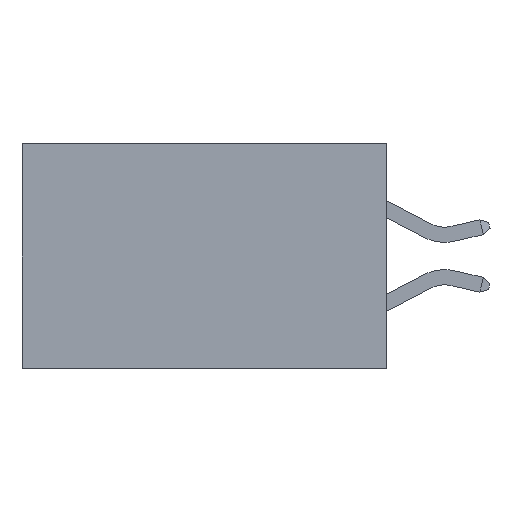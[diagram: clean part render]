
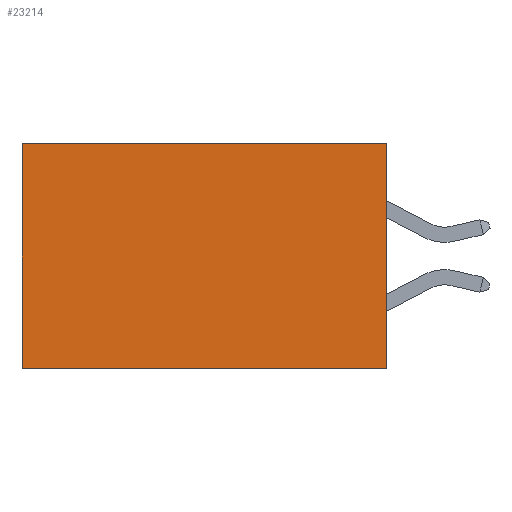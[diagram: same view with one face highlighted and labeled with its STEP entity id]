
A CAD part, left-side view. The second image highlights one B-rep face of the part: STEP entity #23214.
In plain terms, the highlighted planar face has unit normal (-1, 0, 0).
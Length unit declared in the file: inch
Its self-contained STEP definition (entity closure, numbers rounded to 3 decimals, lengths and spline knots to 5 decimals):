
#8 = CARTESIAN_POINT ( 'NONE',  ( 0.2615, 0.6, 0. ) ) ;
#512 = EDGE_CURVE ( 'NONE', #2261, #23418, #26246, .T. ) ;
#736 = DIRECTION ( 'NONE',  ( 0., 0., -1. ) ) ;
#1049 = ORIENTED_EDGE ( 'NONE', *, *, #23925, .T. ) ;
#1179 = ORIENTED_EDGE ( 'NONE', *, *, #15550, .T. ) ;
#2261 = VERTEX_POINT ( 'NONE', #14005 ) ;
#2907 = VECTOR ( 'NONE', #22642, 39.37008 ) ;
#3391 = CARTESIAN_POINT ( 'NONE',  ( 0.2615, 0.6, -0.37 ) ) ;
#4437 = CARTESIAN_POINT ( 'NONE',  ( 0.2615, 0., -0.37 ) ) ;
#4518 = CARTESIAN_POINT ( 'NONE',  ( 0.2615, 0., -0.37 ) ) ;
#5693 = EDGE_CURVE ( 'NONE', #11454, #2261, #9835, .T. ) ;
#6602 = DIRECTION ( 'NONE',  ( 0., 0., -1. ) ) ;
#8144 = VECTOR ( 'NONE', #21657, 39.37008 ) ;
#9596 = VECTOR ( 'NONE', #12702, 39.37008 ) ;
#9835 = LINE ( 'NONE', #4437, #14588 ) ;
#10868 = VERTEX_POINT ( 'NONE', #8 ) ;
#11454 = VERTEX_POINT ( 'NONE', #26179 ) ;
#12702 = DIRECTION ( 'NONE',  ( 0., 1., 0. ) ) ;
#13199 = DIRECTION ( 'NONE',  ( 1., 0., 0. ) ) ;
#13914 = LINE ( 'NONE', #20585, #2907 ) ;
#14005 = CARTESIAN_POINT ( 'NONE',  ( 0.2615, 0., -0.37 ) ) ;
#14588 = VECTOR ( 'NONE', #6602, 39.37008 ) ;
#15148 = PLANE ( 'NONE',  #22758 ) ;
#15550 = EDGE_CURVE ( 'NONE', #11454, #10868, #13914, .T. ) ;
#17703 = ORIENTED_EDGE ( 'NONE', *, *, #5693, .F. ) ;
#18888 = EDGE_LOOP ( 'NONE', ( #1049, #23483, #17703, #1179 ) ) ;
#19605 = CARTESIAN_POINT ( 'NONE',  ( 0.2615, 0.6, -0.37 ) ) ;
#20585 = CARTESIAN_POINT ( 'NONE',  ( 0.2615, 0., 0. ) ) ;
#21657 = DIRECTION ( 'NONE',  ( 0., 0., -1. ) ) ;
#22642 = DIRECTION ( 'NONE',  ( 0., 1., 0. ) ) ;
#22758 = AXIS2_PLACEMENT_3D ( 'NONE', #25232, #13199, #736 ) ;
#23214 = ADVANCED_FACE ( 'NONE', ( #24601 ), #15148, .F. ) ;
#23418 = VERTEX_POINT ( 'NONE', #3391 ) ;
#23483 = ORIENTED_EDGE ( 'NONE', *, *, #512, .F. ) ;
#23925 = EDGE_CURVE ( 'NONE', #10868, #23418, #24230, .T. ) ;
#24230 = LINE ( 'NONE', #19605, #8144 ) ;
#24601 = FACE_OUTER_BOUND ( 'NONE', #18888, .T. ) ;
#25232 = CARTESIAN_POINT ( 'NONE',  ( 0.2615, 0., -0.37 ) ) ;
#26179 = CARTESIAN_POINT ( 'NONE',  ( 0.2615, 0., 0. ) ) ;
#26246 = LINE ( 'NONE', #4518, #9596 ) ;
